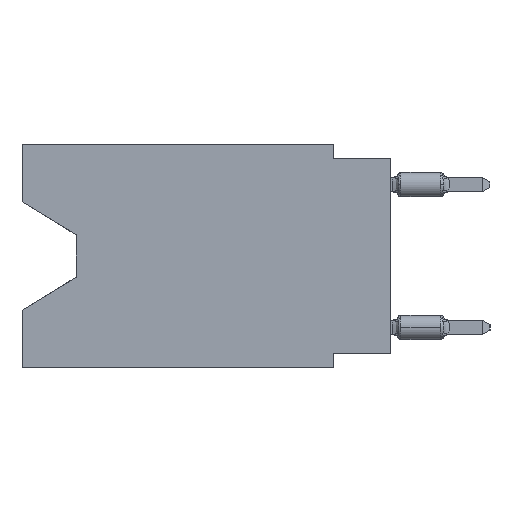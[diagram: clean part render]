
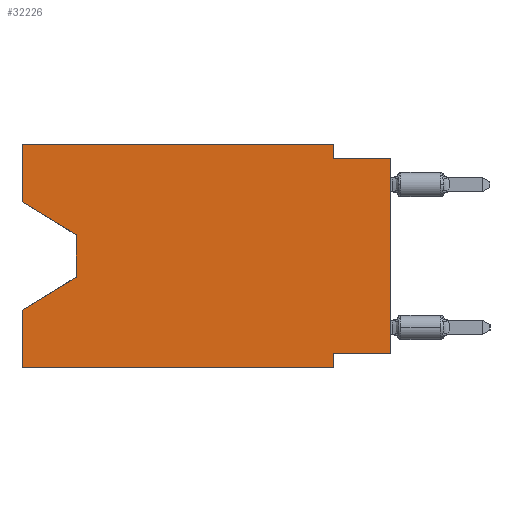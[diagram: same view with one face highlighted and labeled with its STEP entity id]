
A CAD part, left-side view. The second image highlights one B-rep face of the part: STEP entity #32226.
In plain terms, the highlighted planar face has unit normal (-1, 0, 0).
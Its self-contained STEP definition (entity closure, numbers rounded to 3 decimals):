
#708 = PLANE ( 'NONE',  #57641 ) ;
#1794 = LINE ( 'NONE', #19747, #45311 ) ;
#1901 = DIRECTION ( 'NONE',  ( 0., -1., 0. ) ) ;
#2057 = ORIENTED_EDGE ( 'NONE', *, *, #29052, .T. ) ;
#2412 = VERTEX_POINT ( 'NONE', #10489 ) ;
#3011 = VERTEX_POINT ( 'NONE', #48900 ) ;
#3206 = EDGE_LOOP ( 'NONE', ( #36498, #57620, #2057, #30090, #47335, #20929, #40632, #49241, #26603, #28375, #45226, #56770 ) ) ;
#3555 = CARTESIAN_POINT ( 'NONE',  ( 0., 0., -9.271 ) ) ;
#4197 = VECTOR ( 'NONE', #11288, 1000. ) ;
#5117 = DIRECTION ( 'NONE',  ( 0., 0., 1. ) ) ;
#5175 = VECTOR ( 'NONE', #34091, 1000. ) ;
#5375 = VERTEX_POINT ( 'NONE', #29228 ) ;
#5934 = VECTOR ( 'NONE', #43188, 1000. ) ;
#6262 = CARTESIAN_POINT ( 'NONE',  ( 0., 2.54, -0.635 ) ) ;
#7288 = LINE ( 'NONE', #11784, #25073 ) ;
#8809 = FACE_OUTER_BOUND ( 'NONE', #3206, .T. ) ;
#9599 = LINE ( 'NONE', #27891, #44175 ) ;
#9600 = CARTESIAN_POINT ( 'NONE',  ( 0., 16.383, -7.36 ) ) ;
#9862 = VERTEX_POINT ( 'NONE', #16337 ) ;
#10067 = EDGE_CURVE ( 'NONE', #47188, #50320, #38770, .T. ) ;
#10433 = VERTEX_POINT ( 'NONE', #56096 ) ;
#10489 = CARTESIAN_POINT ( 'NONE',  ( 0., 16.383, 0. ) ) ;
#11288 = DIRECTION ( 'NONE',  ( 0., 0., -1. ) ) ;
#11357 = DIRECTION ( 'NONE',  ( 0., -1., 0. ) ) ;
#11784 = CARTESIAN_POINT ( 'NONE',  ( 0., 16.383, -9.906 ) ) ;
#12190 = LINE ( 'NONE', #21183, #5175 ) ;
#13925 = VERTEX_POINT ( 'NONE', #22376 ) ;
#14475 = CARTESIAN_POINT ( 'NONE',  ( 0., 16.383, 0. ) ) ;
#16337 = CARTESIAN_POINT ( 'NONE',  ( 0., 2.54, 0. ) ) ;
#16385 = CARTESIAN_POINT ( 'NONE',  ( 0., 0., -9.271 ) ) ;
#16467 = CARTESIAN_POINT ( 'NONE',  ( 0., 16.383, -2.546 ) ) ;
#16940 = VERTEX_POINT ( 'NONE', #9600 ) ;
#19747 = CARTESIAN_POINT ( 'NONE',  ( 0., 0., -0.635 ) ) ;
#20929 = ORIENTED_EDGE ( 'NONE', *, *, #35719, .F. ) ;
#21088 = DIRECTION ( 'NONE',  ( 0., 0., 1. ) ) ;
#21183 = CARTESIAN_POINT ( 'NONE',  ( 0., 2.54, 0. ) ) ;
#22373 = EDGE_CURVE ( 'NONE', #33086, #3011, #7288, .T. ) ;
#22376 = CARTESIAN_POINT ( 'NONE',  ( 0., 2.54, -9.271 ) ) ;
#22446 = VECTOR ( 'NONE', #33508, 1000. ) ;
#24517 = CARTESIAN_POINT ( 'NONE',  ( 0., 16.383, -9.906 ) ) ;
#25073 = VECTOR ( 'NONE', #52585, 1000. ) ;
#26025 = VECTOR ( 'NONE', #39969, 1000. ) ;
#26331 = DIRECTION ( 'NONE',  ( 0., 0.855, -0.519 ) ) ;
#26603 = ORIENTED_EDGE ( 'NONE', *, *, #35290, .F. ) ;
#27106 = DIRECTION ( 'NONE',  ( 0., 0., -1. ) ) ;
#27891 = CARTESIAN_POINT ( 'NONE',  ( 0., 16.383, 0. ) ) ;
#28375 = ORIENTED_EDGE ( 'NONE', *, *, #38868, .F. ) ;
#28952 = VERTEX_POINT ( 'NONE', #6262 ) ;
#29052 = EDGE_CURVE ( 'NONE', #50320, #16940, #35341, .T. ) ;
#29056 = VERTEX_POINT ( 'NONE', #3555 ) ;
#29228 = CARTESIAN_POINT ( 'NONE',  ( 0., 16.383, -2.546 ) ) ;
#29462 = LINE ( 'NONE', #47457, #30347 ) ;
#29582 = VECTOR ( 'NONE', #21088, 1000. ) ;
#29800 = EDGE_CURVE ( 'NONE', #29056, #10433, #31806, .T. ) ;
#30090 = ORIENTED_EDGE ( 'NONE', *, *, #48383, .F. ) ;
#30347 = VECTOR ( 'NONE', #1901, 1000. ) ;
#31434 = CARTESIAN_POINT ( 'NONE',  ( 0., 13.97, -5.893 ) ) ;
#31615 = CARTESIAN_POINT ( 'NONE',  ( 0., 16.383, 0. ) ) ;
#31806 = LINE ( 'NONE', #43893, #29582 ) ;
#31911 = LINE ( 'NONE', #31615, #41022 ) ;
#32226 = ADVANCED_FACE ( 'NONE', ( #8809 ), #708, .F. ) ;
#33086 = VERTEX_POINT ( 'NONE', #24517 ) ;
#33508 = DIRECTION ( 'NONE',  ( 0., 1., 0. ) ) ;
#33792 = LINE ( 'NONE', #47576, #4197 ) ;
#34091 = DIRECTION ( 'NONE',  ( 0., 0., -1. ) ) ;
#34183 = LINE ( 'NONE', #16467, #5934 ) ;
#35290 = EDGE_CURVE ( 'NONE', #28952, #10433, #1794, .T. ) ;
#35341 = LINE ( 'NONE', #31434, #54465 ) ;
#35719 = EDGE_CURVE ( 'NONE', #13925, #3011, #33792, .T. ) ;
#36498 = ORIENTED_EDGE ( 'NONE', *, *, #50957, .T. ) ;
#36819 = EDGE_CURVE ( 'NONE', #29056, #13925, #47588, .T. ) ;
#38770 = LINE ( 'NONE', #52569, #26025 ) ;
#38868 = EDGE_CURVE ( 'NONE', #9862, #28952, #12190, .T. ) ;
#39969 = DIRECTION ( 'NONE',  ( 0., 0., -1. ) ) ;
#40632 = ORIENTED_EDGE ( 'NONE', *, *, #36819, .F. ) ;
#41022 = VECTOR ( 'NONE', #49898, 1000. ) ;
#41054 = EDGE_CURVE ( 'NONE', #2412, #9862, #29462, .T. ) ;
#42651 = CARTESIAN_POINT ( 'NONE',  ( 0., 13.97, -5.893 ) ) ;
#43188 = DIRECTION ( 'NONE',  ( 0., -0.855, -0.519 ) ) ;
#43893 = CARTESIAN_POINT ( 'NONE',  ( 0., 0., 0. ) ) ;
#44175 = VECTOR ( 'NONE', #5117, 1000. ) ;
#44406 = EDGE_CURVE ( 'NONE', #5375, #2412, #31911, .T. ) ;
#45226 = ORIENTED_EDGE ( 'NONE', *, *, #41054, .F. ) ;
#45311 = VECTOR ( 'NONE', #11357, 1000. ) ;
#47188 = VERTEX_POINT ( 'NONE', #57464 ) ;
#47335 = ORIENTED_EDGE ( 'NONE', *, *, #22373, .T. ) ;
#47457 = CARTESIAN_POINT ( 'NONE',  ( 0., 16.383, 0. ) ) ;
#47576 = CARTESIAN_POINT ( 'NONE',  ( 0., 2.54, -9.906 ) ) ;
#47588 = LINE ( 'NONE', #16385, #22446 ) ;
#48383 = EDGE_CURVE ( 'NONE', #33086, #16940, #9599, .T. ) ;
#48900 = CARTESIAN_POINT ( 'NONE',  ( 0., 2.54, -9.906 ) ) ;
#49241 = ORIENTED_EDGE ( 'NONE', *, *, #29800, .T. ) ;
#49898 = DIRECTION ( 'NONE',  ( 0., 0., 1. ) ) ;
#50320 = VERTEX_POINT ( 'NONE', #42651 ) ;
#50957 = EDGE_CURVE ( 'NONE', #5375, #47188, #34183, .T. ) ;
#52569 = CARTESIAN_POINT ( 'NONE',  ( 0., 13.97, -4.013 ) ) ;
#52585 = DIRECTION ( 'NONE',  ( 0., -1., 0. ) ) ;
#54465 = VECTOR ( 'NONE', #26331, 1000. ) ;
#54979 = DIRECTION ( 'NONE',  ( 1., 0., 0. ) ) ;
#56096 = CARTESIAN_POINT ( 'NONE',  ( 0., 0., -0.635 ) ) ;
#56770 = ORIENTED_EDGE ( 'NONE', *, *, #44406, .F. ) ;
#57464 = CARTESIAN_POINT ( 'NONE',  ( 0., 13.97, -4.013 ) ) ;
#57620 = ORIENTED_EDGE ( 'NONE', *, *, #10067, .T. ) ;
#57641 = AXIS2_PLACEMENT_3D ( 'NONE', #14475, #54979, #27106 ) ;
